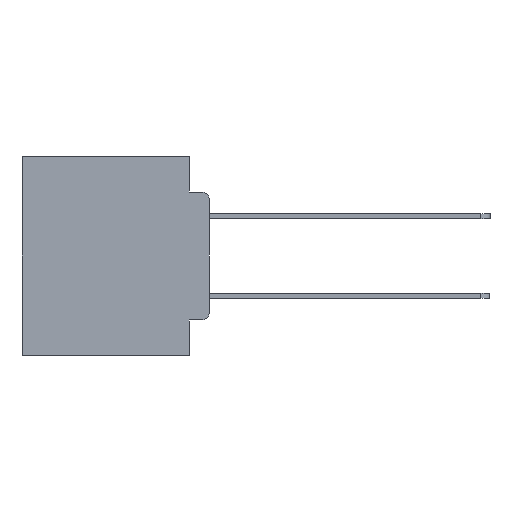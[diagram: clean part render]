
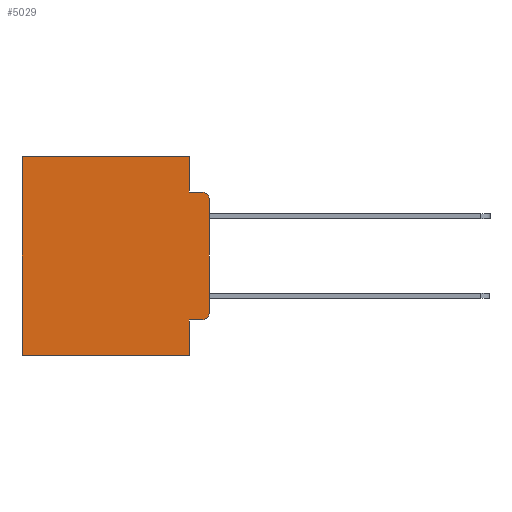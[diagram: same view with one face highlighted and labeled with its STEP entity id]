
A CAD part, left-side view. The second image highlights one B-rep face of the part: STEP entity #5029.
In plain terms, the highlighted planar face has unit normal (-1, 0, 0).
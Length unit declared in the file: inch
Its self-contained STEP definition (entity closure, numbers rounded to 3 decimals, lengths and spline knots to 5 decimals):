
#81 = ORIENTED_EDGE ( 'NONE', *, *, #7429, .F. ) ;
#95 = CARTESIAN_POINT ( 'NONE',  ( 0.298, 0.051, 0. ) ) ;
#147 = ORIENTED_EDGE ( 'NONE', *, *, #12768, .F. ) ;
#427 = ORIENTED_EDGE ( 'NONE', *, *, #22158, .T. ) ;
#455 = ORIENTED_EDGE ( 'NONE', *, *, #23116, .T. ) ;
#721 = ORIENTED_EDGE ( 'NONE', *, *, #767, .F. ) ;
#767 = EDGE_CURVE ( 'NONE', #2177, #8488, #20454, .T. ) ;
#1453 = ORIENTED_EDGE ( 'NONE', *, *, #8140, .T. ) ;
#1803 = DIRECTION ( 'NONE',  ( 0., 1., 0. ) ) ;
#1817 = VECTOR ( 'NONE', #18530, 39.37008 ) ;
#1860 = VERTEX_POINT ( 'NONE', #17819 ) ;
#1998 = CARTESIAN_POINT ( 'NONE',  ( 0.298, 0.473, 0. ) ) ;
#2107 = DIRECTION ( 'NONE',  ( 0., -1., 0. ) ) ;
#2177 = VERTEX_POINT ( 'NONE', #25254 ) ;
#2196 = VERTEX_POINT ( 'NONE', #26024 ) ;
#2202 = ORIENTED_EDGE ( 'NONE', *, *, #11334, .T. ) ;
#2212 = ORIENTED_EDGE ( 'NONE', *, *, #21828, .T. ) ;
#2430 = FACE_OUTER_BOUND ( 'NONE', #23310, .T. ) ;
#2484 = VECTOR ( 'NONE', #2107, 39.37008 ) ;
#2535 = LINE ( 'NONE', #22460, #1817 ) ;
#3866 = CARTESIAN_POINT ( 'NONE',  ( 0.298, 0., 0. ) ) ;
#3967 = EDGE_CURVE ( 'NONE', #15577, #1860, #24528, .T. ) ;
#4163 = DIRECTION ( 'NONE',  ( -1., 0., 0. ) ) ;
#5029 = ADVANCED_FACE ( 'NONE', ( #2430 ), #22058, .F. ) ;
#5595 = DIRECTION ( 'NONE',  ( 0., 1., 0. ) ) ;
#6421 = DIRECTION ( 'NONE',  ( -1., 0., 0. ) ) ;
#7103 = DIRECTION ( 'NONE',  ( 1., 0., 0. ) ) ;
#7136 = DIRECTION ( 'NONE',  ( 0., 0., -1. ) ) ;
#7429 = EDGE_CURVE ( 'NONE', #7767, #15577, #24008, .T. ) ;
#7491 = CARTESIAN_POINT ( 'NONE',  ( 0.298, 0.473, 0. ) ) ;
#7507 = CIRCLE ( 'NONE', #18315, 0.02 ) ;
#7514 = CARTESIAN_POINT ( 'NONE',  ( 0.298, 0., 0. ) ) ;
#7767 = VERTEX_POINT ( 'NONE', #95 ) ;
#8140 = EDGE_CURVE ( 'NONE', #17228, #1860, #12536, .T. ) ;
#8488 = VERTEX_POINT ( 'NONE', #18803 ) ;
#9549 = VERTEX_POINT ( 'NONE', #1998 ) ;
#9748 = VECTOR ( 'NONE', #23334, 39.37008 ) ;
#9792 = DIRECTION ( 'NONE',  ( 0., 0., -1. ) ) ;
#9960 = CARTESIAN_POINT ( 'NONE',  ( 0.298, 0., -0.1085 ) ) ;
#10153 = VECTOR ( 'NONE', #21607, 39.37008 ) ;
#10524 = VERTEX_POINT ( 'NONE', #19359 ) ;
#11245 = ORIENTED_EDGE ( 'NONE', *, *, #18948, .F. ) ;
#11334 = EDGE_CURVE ( 'NONE', #7767, #9549, #22621, .T. ) ;
#11671 = CARTESIAN_POINT ( 'NONE',  ( 0.298, 0., 0. ) ) ;
#11889 = ORIENTED_EDGE ( 'NONE', *, *, #3967, .F. ) ;
#12536 = CIRCLE ( 'NONE', #26203, 0.02 ) ;
#12642 = DIRECTION ( 'NONE',  ( 0., 0., -1. ) ) ;
#12768 = EDGE_CURVE ( 'NONE', #8488, #2196, #24127, .T. ) ;
#13044 = VECTOR ( 'NONE', #5595, 39.37008 ) ;
#13725 = CARTESIAN_POINT ( 'NONE',  ( 0.298, 0., -0.5 ) ) ;
#14006 = AXIS2_PLACEMENT_3D ( 'NONE', #11671, #7103, #7136 ) ;
#14808 = LINE ( 'NONE', #7491, #15422 ) ;
#15422 = VECTOR ( 'NONE', #19550, 39.37008 ) ;
#15567 = LINE ( 'NONE', #7514, #10153 ) ;
#15577 = VERTEX_POINT ( 'NONE', #18500 ) ;
#15591 = CARTESIAN_POINT ( 'NONE',  ( 0.298, 0.02, -0.1085 ) ) ;
#15592 = VERTEX_POINT ( 'NONE', #20515 ) ;
#16188 = CARTESIAN_POINT ( 'NONE',  ( 0.298, 0.051, 0. ) ) ;
#17228 = VERTEX_POINT ( 'NONE', #9960 ) ;
#17410 = VECTOR ( 'NONE', #1803, 39.37008 ) ;
#17819 = CARTESIAN_POINT ( 'NONE',  ( 0.298, 0.02, -0.0885 ) ) ;
#18193 = CARTESIAN_POINT ( 'NONE',  ( 0.298, 0.051, 0. ) ) ;
#18315 = AXIS2_PLACEMENT_3D ( 'NONE', #18504, #6421, #20520 ) ;
#18500 = CARTESIAN_POINT ( 'NONE',  ( 0.298, 0.051, -0.0885 ) ) ;
#18504 = CARTESIAN_POINT ( 'NONE',  ( 0.298, 0.02, -0.3915 ) ) ;
#18530 = DIRECTION ( 'NONE',  ( 0., -1., 0. ) ) ;
#18577 = CARTESIAN_POINT ( 'NONE',  ( 0.298, 0.051, -0.0885 ) ) ;
#18803 = CARTESIAN_POINT ( 'NONE',  ( 0.298, 0.051, -0.5 ) ) ;
#18829 = VECTOR ( 'NONE', #9792, 39.37008 ) ;
#18948 = EDGE_CURVE ( 'NONE', #17228, #15592, #15567, .T. ) ;
#19359 = CARTESIAN_POINT ( 'NONE',  ( 0.298, 0.02, -0.4115 ) ) ;
#19550 = DIRECTION ( 'NONE',  ( 0., 0., -1. ) ) ;
#20454 = LINE ( 'NONE', #18193, #9748 ) ;
#20515 = CARTESIAN_POINT ( 'NONE',  ( 0.298, 0., -0.3915 ) ) ;
#20520 = DIRECTION ( 'NONE',  ( 0., 0., -1. ) ) ;
#21607 = DIRECTION ( 'NONE',  ( 0., 0., -1. ) ) ;
#21828 = EDGE_CURVE ( 'NONE', #10524, #15592, #7507, .T. ) ;
#22058 = PLANE ( 'NONE',  #14006 ) ;
#22158 = EDGE_CURVE ( 'NONE', #9549, #2196, #14808, .T. ) ;
#22460 = CARTESIAN_POINT ( 'NONE',  ( 0.298, 0.051, -0.4115 ) ) ;
#22621 = LINE ( 'NONE', #3866, #17410 ) ;
#23116 = EDGE_CURVE ( 'NONE', #2177, #10524, #2535, .T. ) ;
#23310 = EDGE_LOOP ( 'NONE', ( #11245, #1453, #11889, #81, #2202, #427, #147, #721, #455, #2212 ) ) ;
#23334 = DIRECTION ( 'NONE',  ( 0., 0., -1. ) ) ;
#24008 = LINE ( 'NONE', #16188, #18829 ) ;
#24127 = LINE ( 'NONE', #13725, #13044 ) ;
#24528 = LINE ( 'NONE', #18577, #2484 ) ;
#25254 = CARTESIAN_POINT ( 'NONE',  ( 0.298, 0.051, -0.4115 ) ) ;
#26024 = CARTESIAN_POINT ( 'NONE',  ( 0.298, 0.473, -0.5 ) ) ;
#26203 = AXIS2_PLACEMENT_3D ( 'NONE', #15591, #4163, #12642 ) ;
